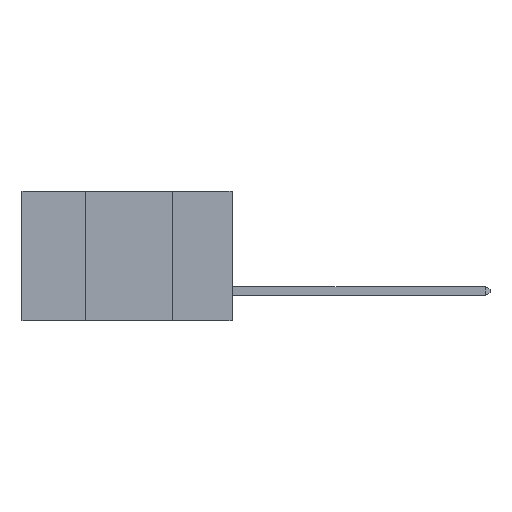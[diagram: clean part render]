
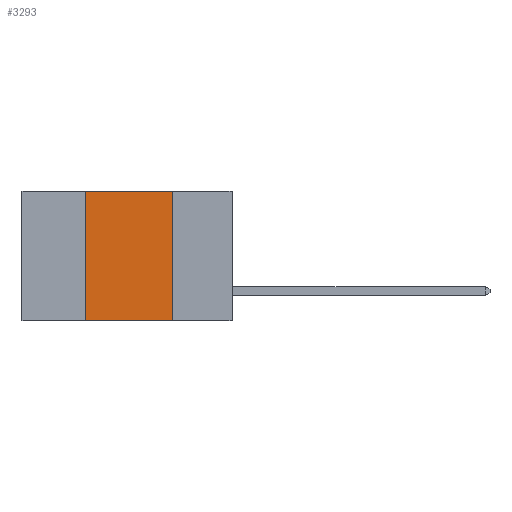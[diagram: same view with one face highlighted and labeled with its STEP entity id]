
A CAD part, left-side view. The second image highlights one B-rep face of the part: STEP entity #3293.
In plain terms, the highlighted planar face has unit normal (-1, 0, 0).
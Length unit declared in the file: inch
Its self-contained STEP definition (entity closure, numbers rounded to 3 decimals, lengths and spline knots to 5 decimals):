
#359 = AXIS2_PLACEMENT_3D ( 'NONE', #16559, #5705, #18393 ) ;
#835 = CARTESIAN_POINT ( 'NONE',  ( 0., 0.42, -0.37 ) ) ;
#836 = LINE ( 'NONE', #8097, #6282 ) ;
#859 = ORIENTED_EDGE ( 'NONE', *, *, #18099, .T. ) ;
#1011 = DIRECTION ( 'NONE',  ( 0., 0., 1. ) ) ;
#1933 = CARTESIAN_POINT ( 'NONE',  ( 0., 0.42, 0. ) ) ;
#2225 = CARTESIAN_POINT ( 'NONE',  ( 0., 0.17, -0.37 ) ) ;
#2263 = CARTESIAN_POINT ( 'NONE',  ( 0., 0.6, -0.37 ) ) ;
#2455 = VERTEX_POINT ( 'NONE', #1933 ) ;
#2492 = VERTEX_POINT ( 'NONE', #835 ) ;
#2684 = VERTEX_POINT ( 'NONE', #16670 ) ;
#3293 = ADVANCED_FACE ( 'NONE', ( #11333 ), #3856, .F. ) ;
#3856 = PLANE ( 'NONE',  #359 ) ;
#3867 = LINE ( 'NONE', #13759, #12986 ) ;
#4556 = VERTEX_POINT ( 'NONE', #2225 ) ;
#5705 = DIRECTION ( 'NONE',  ( 1., 0., 0. ) ) ;
#6282 = VECTOR ( 'NONE', #18959, 39.37008 ) ;
#6945 = LINE ( 'NONE', #8370, #20225 ) ;
#7747 = DIRECTION ( 'NONE',  ( 0., -1., 0. ) ) ;
#8097 = CARTESIAN_POINT ( 'NONE',  ( 0., 0.17, 0. ) ) ;
#8370 = CARTESIAN_POINT ( 'NONE',  ( 0., 0.42, 0. ) ) ;
#9912 = EDGE_CURVE ( 'NONE', #2684, #4556, #836, .T. ) ;
#11333 = FACE_OUTER_BOUND ( 'NONE', #13332, .T. ) ;
#11671 = EDGE_CURVE ( 'NONE', #2455, #2684, #3867, .T. ) ;
#12986 = VECTOR ( 'NONE', #15567, 39.37008 ) ;
#13332 = EDGE_LOOP ( 'NONE', ( #17921, #23252, #14818, #859 ) ) ;
#13567 = EDGE_CURVE ( 'NONE', #2492, #2455, #6945, .T. ) ;
#13759 = CARTESIAN_POINT ( 'NONE',  ( 0., 0.6, 0. ) ) ;
#14818 = ORIENTED_EDGE ( 'NONE', *, *, #13567, .F. ) ;
#15567 = DIRECTION ( 'NONE',  ( 0., -1., 0. ) ) ;
#16559 = CARTESIAN_POINT ( 'NONE',  ( 0., 0.6, 0. ) ) ;
#16670 = CARTESIAN_POINT ( 'NONE',  ( 0., 0.17, 0. ) ) ;
#17921 = ORIENTED_EDGE ( 'NONE', *, *, #9912, .F. ) ;
#18099 = EDGE_CURVE ( 'NONE', #2492, #4556, #19292, .T. ) ;
#18393 = DIRECTION ( 'NONE',  ( 0., 0., -1. ) ) ;
#18723 = VECTOR ( 'NONE', #7747, 39.37008 ) ;
#18959 = DIRECTION ( 'NONE',  ( 0., 0., -1. ) ) ;
#19292 = LINE ( 'NONE', #2263, #18723 ) ;
#20225 = VECTOR ( 'NONE', #1011, 39.37008 ) ;
#23252 = ORIENTED_EDGE ( 'NONE', *, *, #11671, .F. ) ;
